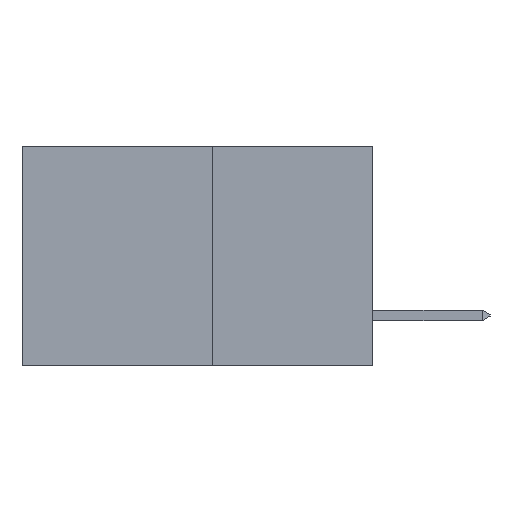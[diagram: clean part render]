
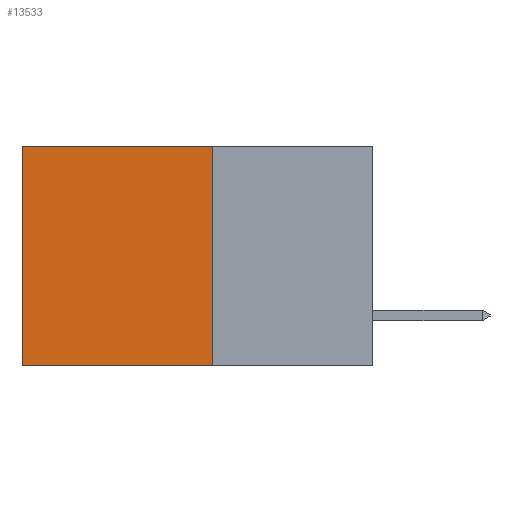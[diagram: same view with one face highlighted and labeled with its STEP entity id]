
A CAD part, left-side view. The second image highlights one B-rep face of the part: STEP entity #13533.
In plain terms, the highlighted planar face has unit normal (-1, 0, 0).
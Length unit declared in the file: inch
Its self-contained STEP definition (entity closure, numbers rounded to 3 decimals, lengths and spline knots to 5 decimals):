
#35 = ORIENTED_EDGE ( 'NONE', *, *, #9257, .F. ) ;
#329 = PLANE ( 'NONE',  #4575 ) ;
#899 = EDGE_CURVE ( 'NONE', #1291, #2615, #2205, .T. ) ;
#1291 = VERTEX_POINT ( 'NONE', #8452 ) ;
#1467 = VERTEX_POINT ( 'NONE', #13554 ) ;
#1535 = DIRECTION ( 'NONE',  ( 1., 0., 0. ) ) ;
#2205 = LINE ( 'NONE', #5944, #5780 ) ;
#2614 = EDGE_LOOP ( 'NONE', ( #14812, #6036, #35, #3647 ) ) ;
#2615 = VERTEX_POINT ( 'NONE', #10392 ) ;
#2813 = CARTESIAN_POINT ( 'NONE',  ( 0.277, 0.59, -0.37 ) ) ;
#3647 = ORIENTED_EDGE ( 'NONE', *, *, #899, .T. ) ;
#4575 = AXIS2_PLACEMENT_3D ( 'NONE', #5142, #1535, #9865 ) ;
#4657 = VERTEX_POINT ( 'NONE', #12650 ) ;
#5142 = CARTESIAN_POINT ( 'NONE',  ( 0.277, 0.27, -0.37 ) ) ;
#5379 = VECTOR ( 'NONE', #5813, 39.37008 ) ;
#5583 = CARTESIAN_POINT ( 'NONE',  ( 0.277, 0.27, -0.37 ) ) ;
#5780 = VECTOR ( 'NONE', #8881, 39.37008 ) ;
#5813 = DIRECTION ( 'NONE',  ( 0., 1., 0. ) ) ;
#5882 = LINE ( 'NONE', #10669, #14653 ) ;
#5944 = CARTESIAN_POINT ( 'NONE',  ( 0.277, 0.27, 0. ) ) ;
#6036 = ORIENTED_EDGE ( 'NONE', *, *, #6865, .F. ) ;
#6572 = LINE ( 'NONE', #2813, #13136 ) ;
#6792 = FACE_OUTER_BOUND ( 'NONE', #2614, .T. ) ;
#6865 = EDGE_CURVE ( 'NONE', #4657, #1467, #11595, .T. ) ;
#8452 = CARTESIAN_POINT ( 'NONE',  ( 0.277, 0.27, 0. ) ) ;
#8881 = DIRECTION ( 'NONE',  ( 0., 1., 0. ) ) ;
#9257 = EDGE_CURVE ( 'NONE', #1291, #4657, #5882, .T. ) ;
#9865 = DIRECTION ( 'NONE',  ( 0., 0., -1. ) ) ;
#10392 = CARTESIAN_POINT ( 'NONE',  ( 0.277, 0.59, 0. ) ) ;
#10669 = CARTESIAN_POINT ( 'NONE',  ( 0.277, 0.27, -0.37 ) ) ;
#10719 = DIRECTION ( 'NONE',  ( 0., 0., -1. ) ) ;
#11060 = DIRECTION ( 'NONE',  ( 0., 0., -1. ) ) ;
#11595 = LINE ( 'NONE', #5583, #5379 ) ;
#12650 = CARTESIAN_POINT ( 'NONE',  ( 0.277, 0.27, -0.37 ) ) ;
#13136 = VECTOR ( 'NONE', #11060, 39.37008 ) ;
#13533 = ADVANCED_FACE ( 'NONE', ( #6792 ), #329, .F. ) ;
#13554 = CARTESIAN_POINT ( 'NONE',  ( 0.277, 0.59, -0.37 ) ) ;
#14140 = EDGE_CURVE ( 'NONE', #2615, #1467, #6572, .T. ) ;
#14653 = VECTOR ( 'NONE', #10719, 39.37008 ) ;
#14812 = ORIENTED_EDGE ( 'NONE', *, *, #14140, .T. ) ;
